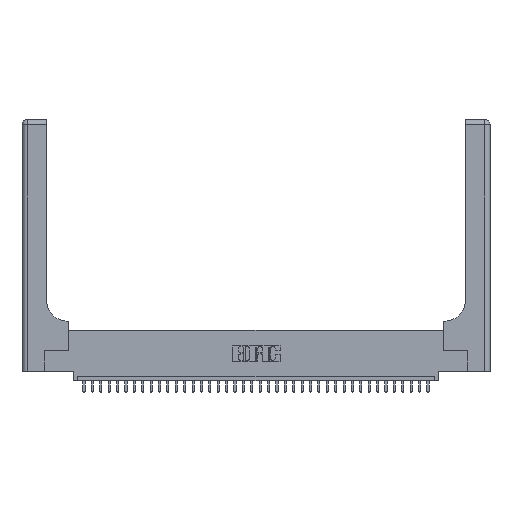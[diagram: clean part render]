
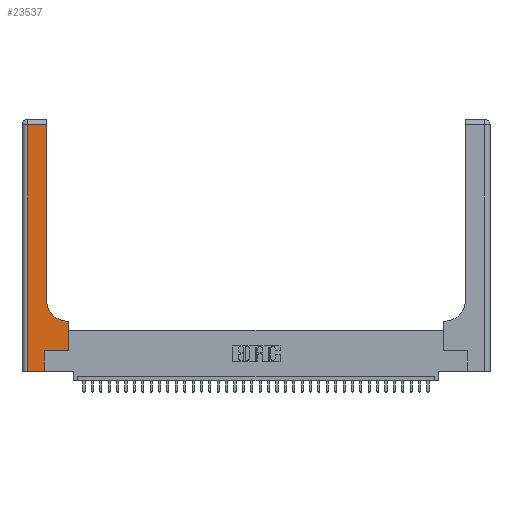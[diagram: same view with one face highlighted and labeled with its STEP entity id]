
A CAD part, top view. The second image highlights one B-rep face of the part: STEP entity #23537.
In plain terms, the highlighted planar face has unit normal (0, 0, 1).
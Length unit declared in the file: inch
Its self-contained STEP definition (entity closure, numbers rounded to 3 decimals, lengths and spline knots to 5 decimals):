
#116 = EDGE_CURVE ( 'NONE', #15052, #6705, #33138, .T. ) ;
#129 = CARTESIAN_POINT ( 'NONE',  ( 0., 3., 0.37 ) ) ;
#1732 = ORIENTED_EDGE ( 'NONE', *, *, #33341, .T. ) ;
#1874 = VERTEX_POINT ( 'NONE', #34288 ) ;
#2030 = CARTESIAN_POINT ( 'NONE',  ( 0.269, 0.25, 0.37 ) ) ;
#2079 = CARTESIAN_POINT ( 'NONE',  ( 0.269, 0., 0.37 ) ) ;
#3313 = CARTESIAN_POINT ( 'NONE',  ( 0.06, 2.94, 0.37 ) ) ;
#4146 = LINE ( 'NONE', #26199, #27809 ) ;
#4363 = FACE_OUTER_BOUND ( 'NONE', #10028, .T. ) ;
#4468 = EDGE_CURVE ( 'NONE', #25550, #33452, #20325, .T. ) ;
#5939 = EDGE_CURVE ( 'NONE', #20345, #36348, #4146, .T. ) ;
#5984 = ORIENTED_EDGE ( 'NONE', *, *, #22742, .T. ) ;
#6150 = CARTESIAN_POINT ( 'NONE',  ( 0.5585, 0.25, 0.37 ) ) ;
#6705 = VERTEX_POINT ( 'NONE', #25356 ) ;
#7368 = AXIS2_PLACEMENT_3D ( 'NONE', #129, #22784, #11582 ) ;
#7774 = DIRECTION ( 'NONE',  ( -1., 0., 0. ) ) ;
#7955 = VERTEX_POINT ( 'NONE', #29248 ) ;
#9754 = ORIENTED_EDGE ( 'NONE', *, *, #4468, .T. ) ;
#9830 = CARTESIAN_POINT ( 'NONE',  ( 0.06, 0., 0.37 ) ) ;
#9963 = LINE ( 'NONE', #2030, #15329 ) ;
#10028 = EDGE_LOOP ( 'NONE', ( #27144, #11207, #24560, #1732, #11127, #10283, #9754, #33362, #5984 ) ) ;
#10141 = LINE ( 'NONE', #30812, #20859 ) ;
#10283 = ORIENTED_EDGE ( 'NONE', *, *, #19706, .T. ) ;
#10454 = CARTESIAN_POINT ( 'NONE',  ( 0.5585, 0.6, 0.37 ) ) ;
#10836 = EDGE_CURVE ( 'NONE', #20453, #7955, #22086, .T. ) ;
#11127 = ORIENTED_EDGE ( 'NONE', *, *, #116, .T. ) ;
#11207 = ORIENTED_EDGE ( 'NONE', *, *, #11300, .T. ) ;
#11300 = EDGE_CURVE ( 'NONE', #7955, #20345, #27508, .T. ) ;
#11582 = DIRECTION ( 'NONE',  ( -1., 0., 0. ) ) ;
#11602 = DIRECTION ( 'NONE',  ( 0., -1., 0. ) ) ;
#15052 = VERTEX_POINT ( 'NONE', #31045 ) ;
#15329 = VECTOR ( 'NONE', #23748, 39.37008 ) ;
#18101 = DIRECTION ( 'NONE',  ( -1., 0., 0. ) ) ;
#19481 = VECTOR ( 'NONE', #7774, 39.37008 ) ;
#19706 = EDGE_CURVE ( 'NONE', #6705, #25550, #9963, .T. ) ;
#20325 = LINE ( 'NONE', #6150, #25227 ) ;
#20345 = VERTEX_POINT ( 'NONE', #3313 ) ;
#20453 = VERTEX_POINT ( 'NONE', #32238 ) ;
#20859 = VECTOR ( 'NONE', #27674, 39.37008 ) ;
#20894 = LINE ( 'NONE', #29575, #35179 ) ;
#22086 = LINE ( 'NONE', #24606, #22976 ) ;
#22742 = EDGE_CURVE ( 'NONE', #1874, #20453, #24423, .T. ) ;
#22784 = DIRECTION ( 'NONE',  ( 0., 0., -1. ) ) ;
#22976 = VECTOR ( 'NONE', #33495, 39.37008 ) ;
#23537 = ADVANCED_FACE ( 'NONE', ( #4363 ), #31307, .F. ) ;
#23748 = DIRECTION ( 'NONE',  ( 1., 0., 0. ) ) ;
#24423 = CIRCLE ( 'NONE', #28636, 0.25 ) ;
#24560 = ORIENTED_EDGE ( 'NONE', *, *, #5939, .T. ) ;
#24606 = CARTESIAN_POINT ( 'NONE',  ( 0.2915, 3., 0.37 ) ) ;
#24835 = DIRECTION ( 'NONE',  ( 0., 1., 0. ) ) ;
#24848 = CARTESIAN_POINT ( 'NONE',  ( 0., 2.94, 0.37 ) ) ;
#25227 = VECTOR ( 'NONE', #31851, 39.37008 ) ;
#25356 = CARTESIAN_POINT ( 'NONE',  ( 0.269, 0.25, 0.37 ) ) ;
#25550 = VERTEX_POINT ( 'NONE', #25726 ) ;
#25726 = CARTESIAN_POINT ( 'NONE',  ( 0.5585, 0.25, 0.37 ) ) ;
#26199 = CARTESIAN_POINT ( 'NONE',  ( 0.06, 3., 0.37 ) ) ;
#27144 = ORIENTED_EDGE ( 'NONE', *, *, #10836, .T. ) ;
#27459 = CARTESIAN_POINT ( 'NONE',  ( 0.5415, 0.85, 0.37 ) ) ;
#27508 = LINE ( 'NONE', #24848, #19481 ) ;
#27674 = DIRECTION ( 'NONE',  ( 1., 0., 0. ) ) ;
#27809 = VECTOR ( 'NONE', #11602, 39.37008 ) ;
#28636 = AXIS2_PLACEMENT_3D ( 'NONE', #27459, #30093, #36057 ) ;
#29248 = CARTESIAN_POINT ( 'NONE',  ( 0.2915, 2.94, 0.37 ) ) ;
#29575 = CARTESIAN_POINT ( 'NONE',  ( 0.2915, 0.6, 0.37 ) ) ;
#30093 = DIRECTION ( 'NONE',  ( 0., 0., -1. ) ) ;
#30812 = CARTESIAN_POINT ( 'NONE',  ( 0., 0., 0.37 ) ) ;
#31045 = CARTESIAN_POINT ( 'NONE',  ( 0.269, 0., 0.37 ) ) ;
#31307 = PLANE ( 'NONE',  #7368 ) ;
#31851 = DIRECTION ( 'NONE',  ( 0., 1., 0. ) ) ;
#32238 = CARTESIAN_POINT ( 'NONE',  ( 0.2915, 0.85, 0.37 ) ) ;
#32241 = VECTOR ( 'NONE', #24835, 39.37008 ) ;
#33119 = EDGE_CURVE ( 'NONE', #33452, #1874, #20894, .T. ) ;
#33138 = LINE ( 'NONE', #2079, #32241 ) ;
#33341 = EDGE_CURVE ( 'NONE', #36348, #15052, #10141, .T. ) ;
#33362 = ORIENTED_EDGE ( 'NONE', *, *, #33119, .T. ) ;
#33452 = VERTEX_POINT ( 'NONE', #10454 ) ;
#33495 = DIRECTION ( 'NONE',  ( 0., 1., 0. ) ) ;
#34288 = CARTESIAN_POINT ( 'NONE',  ( 0.5415, 0.6, 0.37 ) ) ;
#35179 = VECTOR ( 'NONE', #18101, 39.37008 ) ;
#36057 = DIRECTION ( 'NONE',  ( 1., 0., 0. ) ) ;
#36348 = VERTEX_POINT ( 'NONE', #9830 ) ;
